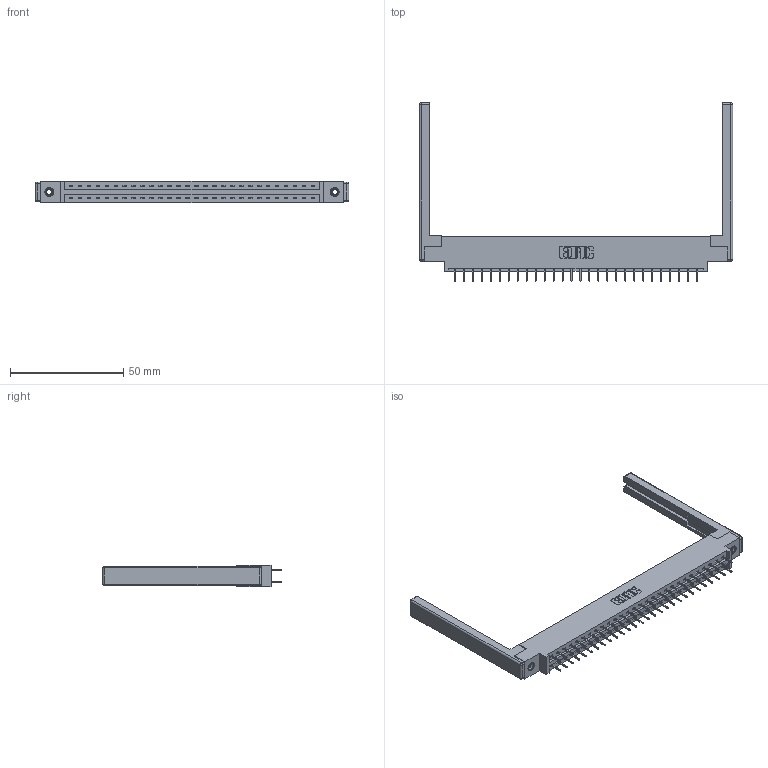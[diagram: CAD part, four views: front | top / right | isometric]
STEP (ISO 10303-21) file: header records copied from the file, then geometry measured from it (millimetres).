
FILE_DESCRIPTION (( 'STEP AP203' ), '1' );
FILE_NAME ('337-056-524-868.STEP', '2019-10-11T19:46:16', ( '' ), ( '' ), 'SwSTEP 2.0', 'SolidWorks 2016', '' );
FILE_SCHEMA (( 'CONFIG_CONTROL_DESIGN' ));
Length unit declared in the file: inch
Products named in the file (5): 345-250-001_345-250-001-102; 337 Part_0.170 Offset - 0.156 Dia-TI; 307-220-068; 337-056-524-868; 345-292-001_345-293-124
Assembly tree (61 placements, depth 2):
  337-056-524-868
    337 Part_0.170 Offset - 0.156 Dia-TI
    345-292-001_345-293-124  x56
    345-250-001_345-250-001-102  x2
    307-220-068  x2
Bounding box: 138.38 x 78.75 x 9.4 mm (x, y, z)
Volume: 18579.7 mm3; surface area: 19791.1 mm2
Topology: 61 solids, 61 shells, 3520 faces, 9953 edges, 6390 vertices
Faces by surface type: plane 2626, cylinder 870, cone 12, sphere 8, torus 4
Entity records: 26486 total; most frequent: CARTESIAN_POINT 4439, ORIENTED_EDGE 4364, DIRECTION 3872, EDGE_CURVE 2182, VECTOR 2008, LINE 2008, VERTEX_POINT 1442, AXIS2_PLACEMENT_3D 932
